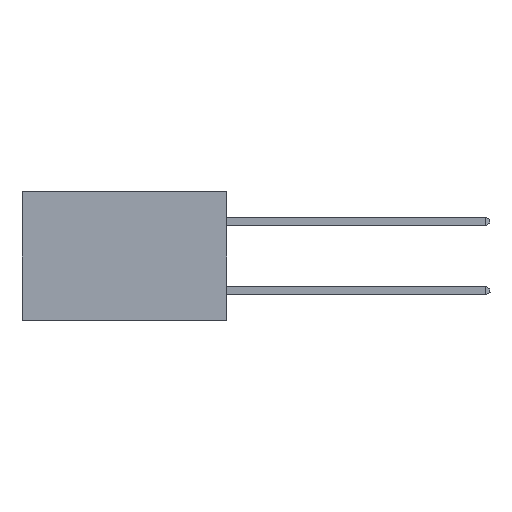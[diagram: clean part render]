
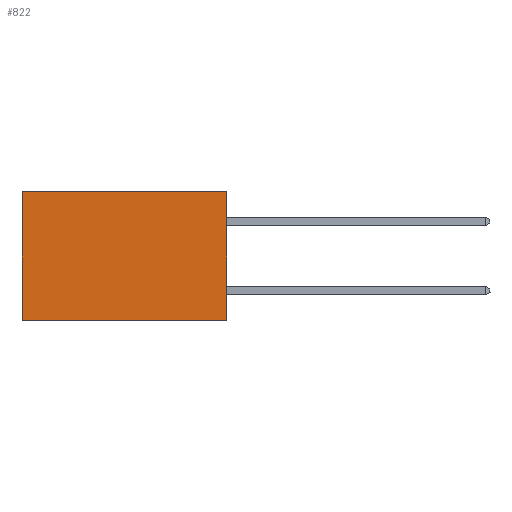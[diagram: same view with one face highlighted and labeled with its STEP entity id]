
A CAD part, left-side view. The second image highlights one B-rep face of the part: STEP entity #822.
In plain terms, the highlighted planar face has unit normal (-1, 0, 0).
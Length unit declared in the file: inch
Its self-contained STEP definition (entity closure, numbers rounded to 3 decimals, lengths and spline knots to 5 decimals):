
#811 = EDGE_LOOP ( 'NONE', ( #17215, #6925, #13945, #7352 ) ) ;
#822 = ADVANCED_FACE ( 'NONE', ( #6438 ), #4084, .F. ) ;
#1950 = CARTESIAN_POINT ( 'NONE',  ( 0.277, 0., -0.37 ) ) ;
#2054 = EDGE_CURVE ( 'NONE', #14503, #25698, #16112, .T. ) ;
#3121 = CARTESIAN_POINT ( 'NONE',  ( 0.277, 0., 0. ) ) ;
#4084 = PLANE ( 'NONE',  #25390 ) ;
#4264 = LINE ( 'NONE', #19164, #15736 ) ;
#5863 = DIRECTION ( 'NONE',  ( 0., 0., -1. ) ) ;
#5996 = DIRECTION ( 'NONE',  ( 1., 0., 0. ) ) ;
#6438 = FACE_OUTER_BOUND ( 'NONE', #811, .T. ) ;
#6550 = EDGE_CURVE ( 'NONE', #23166, #25698, #25385, .T. ) ;
#6925 = ORIENTED_EDGE ( 'NONE', *, *, #6550, .F. ) ;
#7352 = ORIENTED_EDGE ( 'NONE', *, *, #26908, .T. ) ;
#7660 = EDGE_CURVE ( 'NONE', #26546, #23166, #25639, .T. ) ;
#8712 = CARTESIAN_POINT ( 'NONE',  ( 0.277, 0.59, -0.37 ) ) ;
#10619 = DIRECTION ( 'NONE',  ( 0., 1., 0. ) ) ;
#13460 = VECTOR ( 'NONE', #10619, 39.37008 ) ;
#13666 = DIRECTION ( 'NONE',  ( 0., 0., -1. ) ) ;
#13945 = ORIENTED_EDGE ( 'NONE', *, *, #7660, .F. ) ;
#14412 = VECTOR ( 'NONE', #22822, 39.37008 ) ;
#14503 = VERTEX_POINT ( 'NONE', #15937 ) ;
#15736 = VECTOR ( 'NONE', #25469, 39.37008 ) ;
#15937 = CARTESIAN_POINT ( 'NONE',  ( 0.277, 0.59, 0. ) ) ;
#16112 = LINE ( 'NONE', #17258, #16775 ) ;
#16434 = CARTESIAN_POINT ( 'NONE',  ( 0.277, 0., -0.37 ) ) ;
#16498 = CARTESIAN_POINT ( 'NONE',  ( 0.277, 0., -0.37 ) ) ;
#16775 = VECTOR ( 'NONE', #5863, 39.37008 ) ;
#17215 = ORIENTED_EDGE ( 'NONE', *, *, #2054, .T. ) ;
#17258 = CARTESIAN_POINT ( 'NONE',  ( 0.277, 0.59, -0.37 ) ) ;
#19164 = CARTESIAN_POINT ( 'NONE',  ( 0.277, 0., 0. ) ) ;
#22689 = CARTESIAN_POINT ( 'NONE',  ( 0.277, 0., -0.37 ) ) ;
#22822 = DIRECTION ( 'NONE',  ( 0., 0., -1. ) ) ;
#23166 = VERTEX_POINT ( 'NONE', #22689 ) ;
#25385 = LINE ( 'NONE', #1950, #13460 ) ;
#25390 = AXIS2_PLACEMENT_3D ( 'NONE', #16498, #5996, #13666 ) ;
#25469 = DIRECTION ( 'NONE',  ( 0., 1., 0. ) ) ;
#25639 = LINE ( 'NONE', #16434, #14412 ) ;
#25698 = VERTEX_POINT ( 'NONE', #8712 ) ;
#26546 = VERTEX_POINT ( 'NONE', #3121 ) ;
#26908 = EDGE_CURVE ( 'NONE', #26546, #14503, #4264, .T. ) ;
